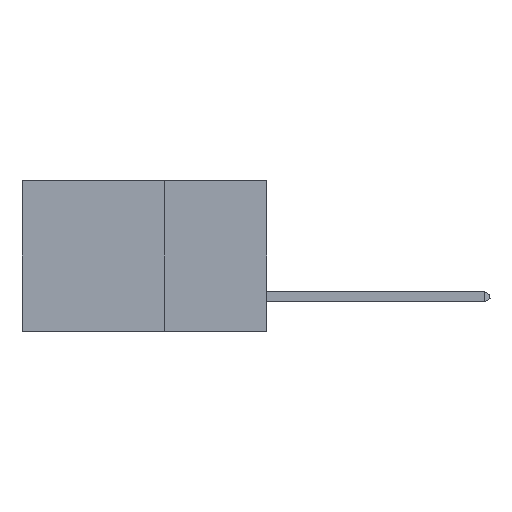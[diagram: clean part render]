
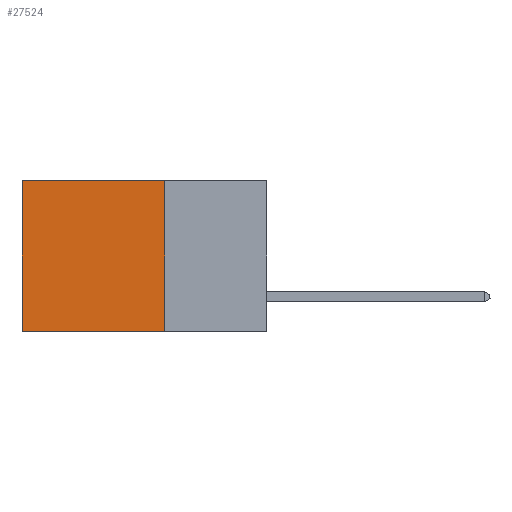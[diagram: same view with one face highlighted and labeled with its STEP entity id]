
A CAD part, left-side view. The second image highlights one B-rep face of the part: STEP entity #27524.
In plain terms, the highlighted planar face has unit normal (-1, 0, 0).
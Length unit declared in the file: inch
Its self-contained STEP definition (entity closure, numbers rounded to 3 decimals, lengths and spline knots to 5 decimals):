
#14 = EDGE_CURVE ( 'NONE', #19010, #33574, #7035, .T. ) ;
#471 = DIRECTION ( 'NONE',  ( 0., 1., 0. ) ) ;
#2137 = DIRECTION ( 'NONE',  ( 0., 1., 0. ) ) ;
#2538 = VECTOR ( 'NONE', #2137, 39.37008 ) ;
#3499 = ORIENTED_EDGE ( 'NONE', *, *, #14, .T. ) ;
#3714 = CARTESIAN_POINT ( 'NONE',  ( 0.2875, 0.6, 0. ) ) ;
#3859 = ORIENTED_EDGE ( 'NONE', *, *, #10409, .F. ) ;
#4916 = FACE_OUTER_BOUND ( 'NONE', #26741, .T. ) ;
#6272 = DIRECTION ( 'NONE',  ( 0., 0., -1. ) ) ;
#6389 = CARTESIAN_POINT ( 'NONE',  ( 0.2875, 0.6, -0.37 ) ) ;
#7035 = LINE ( 'NONE', #29985, #26181 ) ;
#8496 = EDGE_CURVE ( 'NONE', #19010, #39783, #31146, .T. ) ;
#10409 = EDGE_CURVE ( 'NONE', #39783, #24267, #41266, .T. ) ;
#10546 = AXIS2_PLACEMENT_3D ( 'NONE', #38118, #41557, #12151 ) ;
#12151 = DIRECTION ( 'NONE',  ( 0., 0., -1. ) ) ;
#13495 = CARTESIAN_POINT ( 'NONE',  ( 0.2875, 0.6, 0. ) ) ;
#14459 = DIRECTION ( 'NONE',  ( 0., 0., -1. ) ) ;
#15542 = LINE ( 'NONE', #13495, #22255 ) ;
#19010 = VERTEX_POINT ( 'NONE', #31510 ) ;
#19179 = EDGE_CURVE ( 'NONE', #33574, #24267, #15542, .T. ) ;
#19271 = CARTESIAN_POINT ( 'NONE',  ( 0.2875, 0.25, 0. ) ) ;
#19720 = ORIENTED_EDGE ( 'NONE', *, *, #19179, .T. ) ;
#20879 = CARTESIAN_POINT ( 'NONE',  ( 0.2875, 0.25, -0.37 ) ) ;
#22255 = VECTOR ( 'NONE', #14459, 39.37008 ) ;
#24267 = VERTEX_POINT ( 'NONE', #6389 ) ;
#25459 = PLANE ( 'NONE',  #10546 ) ;
#26181 = VECTOR ( 'NONE', #471, 39.37008 ) ;
#26741 = EDGE_LOOP ( 'NONE', ( #19720, #3859, #33166, #3499 ) ) ;
#27524 = ADVANCED_FACE ( 'NONE', ( #4916 ), #25459, .F. ) ;
#29985 = CARTESIAN_POINT ( 'NONE',  ( 0.2875, 0.25, 0. ) ) ;
#31146 = LINE ( 'NONE', #19271, #41903 ) ;
#31510 = CARTESIAN_POINT ( 'NONE',  ( 0.2875, 0.25, 0. ) ) ;
#33166 = ORIENTED_EDGE ( 'NONE', *, *, #8496, .F. ) ;
#33574 = VERTEX_POINT ( 'NONE', #3714 ) ;
#38118 = CARTESIAN_POINT ( 'NONE',  ( 0.2875, 0.25, 0. ) ) ;
#39783 = VERTEX_POINT ( 'NONE', #20879 ) ;
#41261 = CARTESIAN_POINT ( 'NONE',  ( 0.2875, 0.25, -0.37 ) ) ;
#41266 = LINE ( 'NONE', #41261, #2538 ) ;
#41557 = DIRECTION ( 'NONE',  ( 1., 0., 0. ) ) ;
#41903 = VECTOR ( 'NONE', #6272, 39.37008 ) ;
